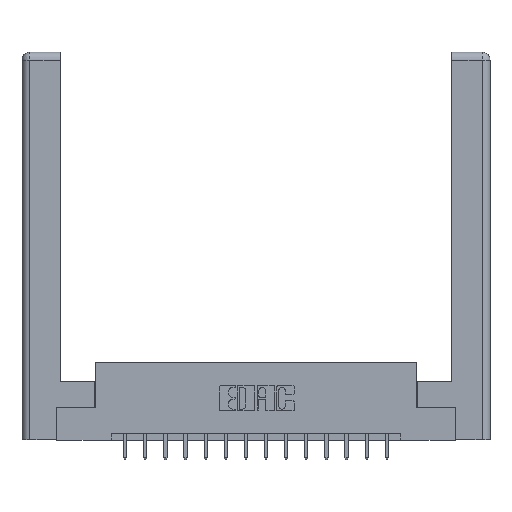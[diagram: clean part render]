
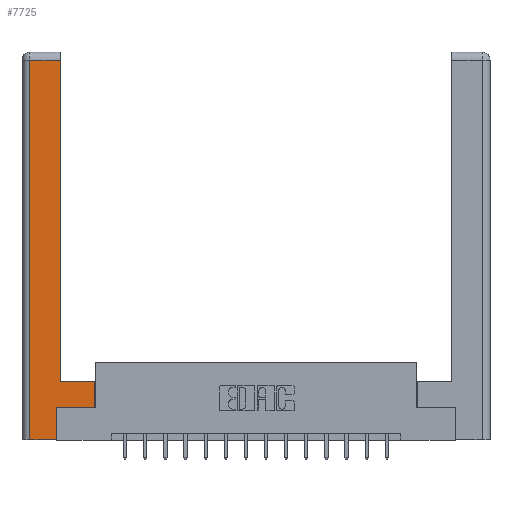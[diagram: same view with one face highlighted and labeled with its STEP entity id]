
A CAD part, top view. The second image highlights one B-rep face of the part: STEP entity #7725.
In plain terms, the highlighted planar face has unit normal (0, 0, 1).
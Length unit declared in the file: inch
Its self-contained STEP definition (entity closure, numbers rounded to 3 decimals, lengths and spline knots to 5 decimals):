
#275 = ORIENTED_EDGE ( 'NONE', *, *, #13262, .T. ) ;
#644 = CARTESIAN_POINT ( 'NONE',  ( 0.295, 3., 0. ) ) ;
#658 = EDGE_CURVE ( 'NONE', #15332, #13725, #12923, .T. ) ;
#856 = DIRECTION ( 'NONE',  ( 0., 1., 0. ) ) ;
#1033 = VERTEX_POINT ( 'NONE', #14206 ) ;
#1061 = LINE ( 'NONE', #10433, #3783 ) ;
#1146 = CARTESIAN_POINT ( 'NONE',  ( 0.0615, 2.94, 0. ) ) ;
#1169 = VERTEX_POINT ( 'NONE', #13582 ) ;
#1253 = DIRECTION ( 'NONE',  ( -1., 0., 0. ) ) ;
#1483 = CARTESIAN_POINT ( 'NONE',  ( 0.295, 0.45, 0. ) ) ;
#1580 = EDGE_CURVE ( 'NONE', #4818, #7271, #4667, .T. ) ;
#1829 = EDGE_CURVE ( 'NONE', #13725, #3413, #15585, .T. ) ;
#1873 = CARTESIAN_POINT ( 'NONE',  ( 0.265, 0., 0. ) ) ;
#2342 = CARTESIAN_POINT ( 'NONE',  ( 0.265, 0.245, 0. ) ) ;
#2767 = LINE ( 'NONE', #1146, #4037 ) ;
#2889 = CARTESIAN_POINT ( 'NONE',  ( 0., 0., 0. ) ) ;
#2908 = CARTESIAN_POINT ( 'NONE',  ( 0.0615, 2.94, 0. ) ) ;
#3012 = VECTOR ( 'NONE', #6699, 39.37008 ) ;
#3204 = ORIENTED_EDGE ( 'NONE', *, *, #658, .T. ) ;
#3413 = VERTEX_POINT ( 'NONE', #3508 ) ;
#3508 = CARTESIAN_POINT ( 'NONE',  ( 0.565, 0.245, 0. ) ) ;
#3783 = VECTOR ( 'NONE', #6541, 39.37008 ) ;
#3867 = LINE ( 'NONE', #16806, #6559 ) ;
#4037 = VECTOR ( 'NONE', #1253, 39.37008 ) ;
#4431 = PLANE ( 'NONE',  #16382 ) ;
#4667 = LINE ( 'NONE', #644, #15605 ) ;
#4692 = LINE ( 'NONE', #15573, #16476 ) ;
#4818 = VERTEX_POINT ( 'NONE', #1483 ) ;
#4915 = CARTESIAN_POINT ( 'NONE',  ( 0.265, 0.245, 0. ) ) ;
#5372 = ORIENTED_EDGE ( 'NONE', *, *, #12665, .T. ) ;
#5447 = EDGE_CURVE ( 'NONE', #5474, #1033, #10669, .T. ) ;
#5468 = DIRECTION ( 'NONE',  ( 1., 0., 0. ) ) ;
#5474 = VERTEX_POINT ( 'NONE', #2908 ) ;
#5700 = ORIENTED_EDGE ( 'NONE', *, *, #12207, .T. ) ;
#5862 = CARTESIAN_POINT ( 'NONE',  ( 0.295, 2.94, 0. ) ) ;
#6060 = DIRECTION ( 'NONE',  ( -1., 0., 0. ) ) ;
#6541 = DIRECTION ( 'NONE',  ( 1., 0., 0. ) ) ;
#6559 = VECTOR ( 'NONE', #6060, 39.37008 ) ;
#6699 = DIRECTION ( 'NONE',  ( 0., -1., 0. ) ) ;
#7136 = VECTOR ( 'NONE', #5468, 39.37008 ) ;
#7271 = VERTEX_POINT ( 'NONE', #5862 ) ;
#7725 = ADVANCED_FACE ( 'NONE', ( #9555 ), #4431, .F. ) ;
#7861 = EDGE_CURVE ( 'NONE', #1033, #15332, #1061, .T. ) ;
#8962 = ORIENTED_EDGE ( 'NONE', *, *, #7861, .T. ) ;
#9555 = FACE_OUTER_BOUND ( 'NONE', #10450, .T. ) ;
#9905 = DIRECTION ( 'NONE',  ( 0., 1., 0. ) ) ;
#10433 = CARTESIAN_POINT ( 'NONE',  ( 0.265, 0., 0. ) ) ;
#10450 = EDGE_LOOP ( 'NONE', ( #11807, #275, #15093, #8962, #3204, #16177, #5372, #5700 ) ) ;
#10669 = LINE ( 'NONE', #12166, #3012 ) ;
#11042 = DIRECTION ( 'NONE',  ( -1., 0., 0. ) ) ;
#11807 = ORIENTED_EDGE ( 'NONE', *, *, #1580, .T. ) ;
#12166 = CARTESIAN_POINT ( 'NONE',  ( 0.0615, 0., 0. ) ) ;
#12207 = EDGE_CURVE ( 'NONE', #1169, #4818, #3867, .T. ) ;
#12665 = EDGE_CURVE ( 'NONE', #3413, #1169, #4692, .T. ) ;
#12923 = LINE ( 'NONE', #4915, #13767 ) ;
#13262 = EDGE_CURVE ( 'NONE', #7271, #5474, #2767, .T. ) ;
#13473 = DIRECTION ( 'NONE',  ( 0., 0., -1. ) ) ;
#13582 = CARTESIAN_POINT ( 'NONE',  ( 0.565, 0.45, 0. ) ) ;
#13597 = CARTESIAN_POINT ( 'NONE',  ( 0.565, 0.245, 0. ) ) ;
#13725 = VERTEX_POINT ( 'NONE', #2342 ) ;
#13767 = VECTOR ( 'NONE', #856, 39.37008 ) ;
#14206 = CARTESIAN_POINT ( 'NONE',  ( 0.0615, 0., 0. ) ) ;
#15093 = ORIENTED_EDGE ( 'NONE', *, *, #5447, .T. ) ;
#15332 = VERTEX_POINT ( 'NONE', #1873 ) ;
#15573 = CARTESIAN_POINT ( 'NONE',  ( 0.565, 0.45, 0. ) ) ;
#15585 = LINE ( 'NONE', #13597, #7136 ) ;
#15605 = VECTOR ( 'NONE', #9905, 39.37008 ) ;
#15637 = DIRECTION ( 'NONE',  ( 0., 1., 0. ) ) ;
#16177 = ORIENTED_EDGE ( 'NONE', *, *, #1829, .T. ) ;
#16382 = AXIS2_PLACEMENT_3D ( 'NONE', #2889, #13473, #11042 ) ;
#16476 = VECTOR ( 'NONE', #15637, 39.37008 ) ;
#16806 = CARTESIAN_POINT ( 'NONE',  ( 0.295, 0.45, 0. ) ) ;
